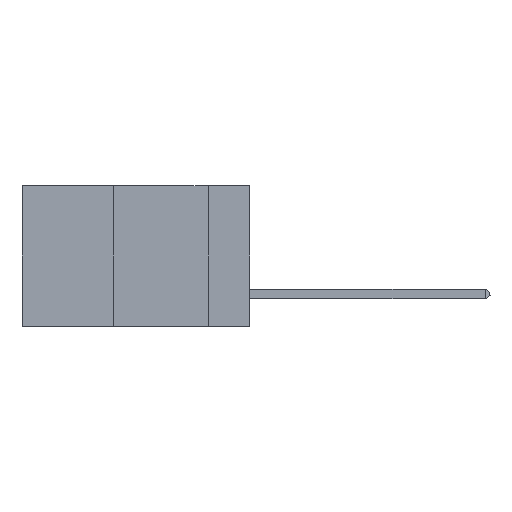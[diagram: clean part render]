
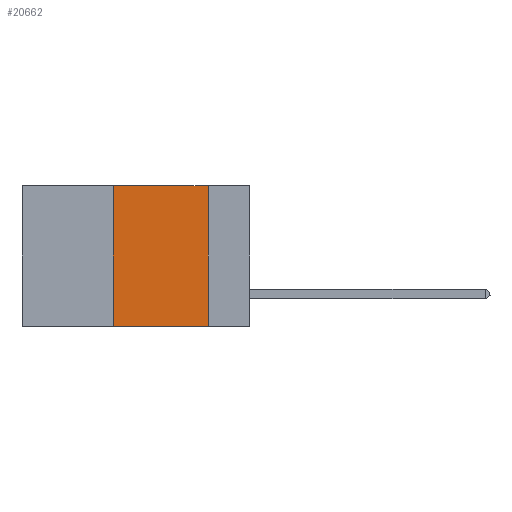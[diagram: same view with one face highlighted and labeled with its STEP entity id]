
A CAD part, left-side view. The second image highlights one B-rep face of the part: STEP entity #20662.
In plain terms, the highlighted planar face has unit normal (-1, 0, 0).
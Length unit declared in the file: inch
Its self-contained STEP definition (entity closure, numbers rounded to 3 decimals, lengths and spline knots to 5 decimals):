
#1009 = CARTESIAN_POINT ( 'NONE',  ( 0., 0.6, -0.37 ) ) ;
#2496 = CARTESIAN_POINT ( 'NONE',  ( 0., 0.11, -0.37 ) ) ;
#3117 = DIRECTION ( 'NONE',  ( 0., -1., 0. ) ) ;
#4303 = DIRECTION ( 'NONE',  ( 1., 0., 0. ) ) ;
#4308 = EDGE_CURVE ( 'NONE', #5687, #23886, #12200, .T. ) ;
#5571 = CARTESIAN_POINT ( 'NONE',  ( 0., 0.6, 0. ) ) ;
#5687 = VERTEX_POINT ( 'NONE', #14684 ) ;
#8005 = EDGE_CURVE ( 'NONE', #17499, #23886, #9360, .T. ) ;
#9142 = VECTOR ( 'NONE', #22051, 39.37008 ) ;
#9360 = LINE ( 'NONE', #13809, #20410 ) ;
#9894 = CARTESIAN_POINT ( 'NONE',  ( 0., 0.36, 0. ) ) ;
#10084 = EDGE_CURVE ( 'NONE', #5687, #21704, #25716, .T. ) ;
#10615 = ORIENTED_EDGE ( 'NONE', *, *, #4308, .T. ) ;
#12083 = CARTESIAN_POINT ( 'NONE',  ( 0., 0.36, 0. ) ) ;
#12114 = CARTESIAN_POINT ( 'NONE',  ( 0., 0.11, 0. ) ) ;
#12200 = LINE ( 'NONE', #1009, #18991 ) ;
#12272 = VECTOR ( 'NONE', #14143, 39.37008 ) ;
#13080 = EDGE_CURVE ( 'NONE', #21704, #17499, #17754, .T. ) ;
#13809 = CARTESIAN_POINT ( 'NONE',  ( 0., 0.11, 0. ) ) ;
#13891 = DIRECTION ( 'NONE',  ( 0., 0., -1. ) ) ;
#14143 = DIRECTION ( 'NONE',  ( 0., -1., 0. ) ) ;
#14684 = CARTESIAN_POINT ( 'NONE',  ( 0., 0.36, -0.37 ) ) ;
#14879 = PLANE ( 'NONE',  #20828 ) ;
#17499 = VERTEX_POINT ( 'NONE', #12114 ) ;
#17593 = ORIENTED_EDGE ( 'NONE', *, *, #13080, .F. ) ;
#17754 = LINE ( 'NONE', #20088, #12272 ) ;
#18945 = EDGE_LOOP ( 'NONE', ( #23054, #17593, #21650, #10615 ) ) ;
#18991 = VECTOR ( 'NONE', #3117, 39.37008 ) ;
#20088 = CARTESIAN_POINT ( 'NONE',  ( 0., 0.6, 0. ) ) ;
#20410 = VECTOR ( 'NONE', #13891, 39.37008 ) ;
#20662 = ADVANCED_FACE ( 'NONE', ( #24440 ), #14879, .F. ) ;
#20828 = AXIS2_PLACEMENT_3D ( 'NONE', #5571, #4303, #20857 ) ;
#20857 = DIRECTION ( 'NONE',  ( 0., 0., -1. ) ) ;
#21650 = ORIENTED_EDGE ( 'NONE', *, *, #10084, .F. ) ;
#21704 = VERTEX_POINT ( 'NONE', #12083 ) ;
#22051 = DIRECTION ( 'NONE',  ( 0., 0., 1. ) ) ;
#23054 = ORIENTED_EDGE ( 'NONE', *, *, #8005, .F. ) ;
#23886 = VERTEX_POINT ( 'NONE', #2496 ) ;
#24440 = FACE_OUTER_BOUND ( 'NONE', #18945, .T. ) ;
#25716 = LINE ( 'NONE', #9894, #9142 ) ;
